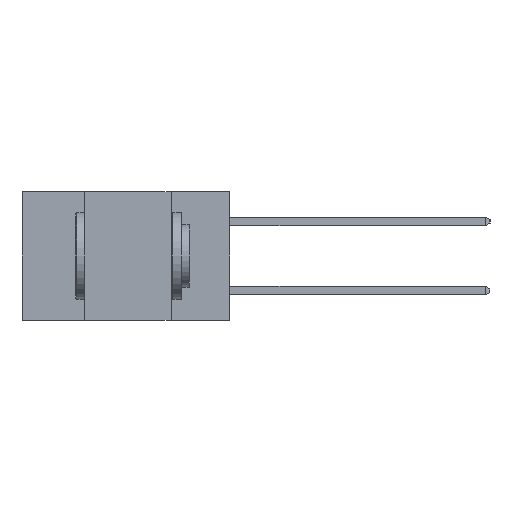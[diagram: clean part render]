
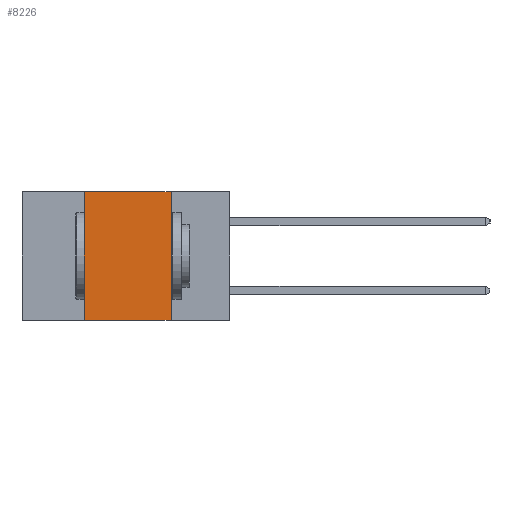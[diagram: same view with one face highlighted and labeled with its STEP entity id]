
A CAD part, left-side view. The second image highlights one B-rep face of the part: STEP entity #8226.
In plain terms, the highlighted planar face has unit normal (-1, 0, 0).
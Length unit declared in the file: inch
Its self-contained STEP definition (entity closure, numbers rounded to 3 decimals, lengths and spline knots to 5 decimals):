
#34 = DIRECTION ( 'NONE',  ( 0., 0., 1. ) ) ;
#432 = CARTESIAN_POINT ( 'NONE',  ( 0., 0.42, 0. ) ) ;
#1165 = VECTOR ( 'NONE', #1872, 39.37008 ) ;
#1204 = DIRECTION ( 'NONE',  ( 0., 0., -1. ) ) ;
#1255 = VERTEX_POINT ( 'NONE', #7230 ) ;
#1436 = VECTOR ( 'NONE', #5021, 39.37008 ) ;
#1534 = CARTESIAN_POINT ( 'NONE',  ( 0., 0.6, 0. ) ) ;
#1872 = DIRECTION ( 'NONE',  ( 0., -1., 0. ) ) ;
#2331 = VERTEX_POINT ( 'NONE', #4879 ) ;
#3225 = EDGE_CURVE ( 'NONE', #6301, #1255, #5192, .T. ) ;
#3288 = LINE ( 'NONE', #9379, #1436 ) ;
#4214 = ORIENTED_EDGE ( 'NONE', *, *, #7400, .T. ) ;
#4553 = EDGE_LOOP ( 'NONE', ( #5949, #9747, #5613, #4214 ) ) ;
#4625 = VECTOR ( 'NONE', #34, 39.37008 ) ;
#4747 = FACE_OUTER_BOUND ( 'NONE', #4553, .T. ) ;
#4868 = LINE ( 'NONE', #432, #4625 ) ;
#4879 = CARTESIAN_POINT ( 'NONE',  ( 0., 0.17, -0.37 ) ) ;
#5021 = DIRECTION ( 'NONE',  ( 0., -1., 0. ) ) ;
#5192 = LINE ( 'NONE', #1534, #1165 ) ;
#5217 = CARTESIAN_POINT ( 'NONE',  ( 0., 0.6, 0. ) ) ;
#5225 = DIRECTION ( 'NONE',  ( 0., 0., -1. ) ) ;
#5358 = VECTOR ( 'NONE', #5225, 39.37008 ) ;
#5501 = AXIS2_PLACEMENT_3D ( 'NONE', #5217, #5965, #1204 ) ;
#5613 = ORIENTED_EDGE ( 'NONE', *, *, #7246, .F. ) ;
#5949 = ORIENTED_EDGE ( 'NONE', *, *, #7158, .F. ) ;
#5965 = DIRECTION ( 'NONE',  ( 1., 0., 0. ) ) ;
#5976 = VERTEX_POINT ( 'NONE', #6572 ) ;
#6301 = VERTEX_POINT ( 'NONE', #8330 ) ;
#6572 = CARTESIAN_POINT ( 'NONE',  ( 0., 0.42, -0.37 ) ) ;
#7158 = EDGE_CURVE ( 'NONE', #1255, #2331, #7266, .T. ) ;
#7230 = CARTESIAN_POINT ( 'NONE',  ( 0., 0.17, 0. ) ) ;
#7246 = EDGE_CURVE ( 'NONE', #5976, #6301, #4868, .T. ) ;
#7266 = LINE ( 'NONE', #9583, #5358 ) ;
#7400 = EDGE_CURVE ( 'NONE', #5976, #2331, #3288, .T. ) ;
#8226 = ADVANCED_FACE ( 'NONE', ( #4747 ), #9558, .F. ) ;
#8330 = CARTESIAN_POINT ( 'NONE',  ( 0., 0.42, 0. ) ) ;
#9379 = CARTESIAN_POINT ( 'NONE',  ( 0., 0.6, -0.37 ) ) ;
#9558 = PLANE ( 'NONE',  #5501 ) ;
#9583 = CARTESIAN_POINT ( 'NONE',  ( 0., 0.17, 0. ) ) ;
#9747 = ORIENTED_EDGE ( 'NONE', *, *, #3225, .F. ) ;
